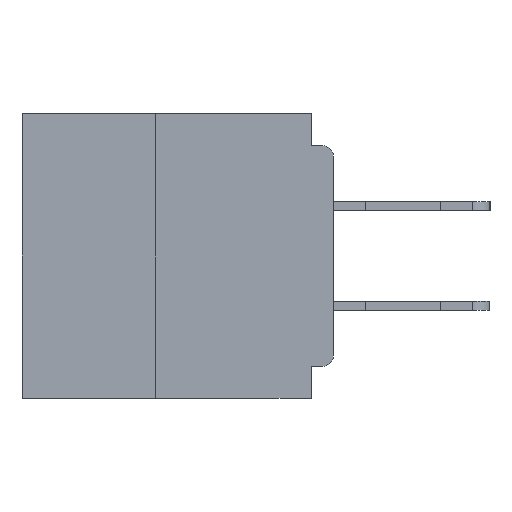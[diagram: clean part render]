
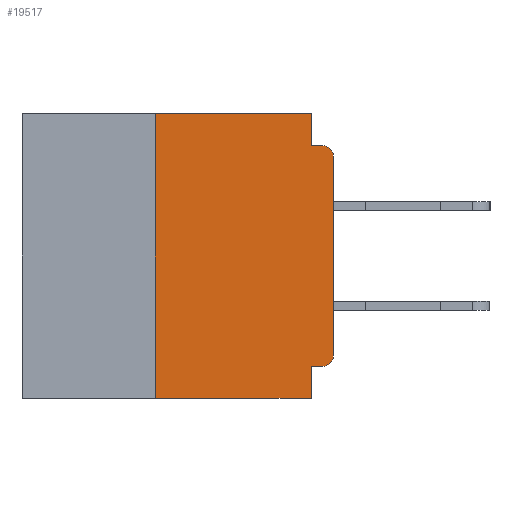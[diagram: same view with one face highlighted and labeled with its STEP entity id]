
A CAD part, left-side view. The second image highlights one B-rep face of the part: STEP entity #19517.
In plain terms, the highlighted planar face has unit normal (-1, 0, 0).
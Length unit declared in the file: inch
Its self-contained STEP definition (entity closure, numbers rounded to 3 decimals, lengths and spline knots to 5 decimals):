
#473 = EDGE_CURVE ( 'NONE', #25092, #37053, #29028, .T. ) ;
#1003 = ORIENTED_EDGE ( 'NONE', *, *, #13540, .F. ) ;
#2314 = VERTEX_POINT ( 'NONE', #25196 ) ;
#2443 = LINE ( 'NONE', #6597, #16447 ) ;
#2663 = EDGE_CURVE ( 'NONE', #30308, #9962, #35684, .T. ) ;
#3345 = DIRECTION ( 'NONE',  ( 0., 0., -1. ) ) ;
#3607 = ORIENTED_EDGE ( 'NONE', *, *, #13655, .T. ) ;
#4194 = VECTOR ( 'NONE', #34065, 39.37008 ) ;
#6597 = CARTESIAN_POINT ( 'NONE',  ( 0., 0.031, 0. ) ) ;
#7806 = CARTESIAN_POINT ( 'NONE',  ( 0., 0.25, -0.4 ) ) ;
#8055 = DIRECTION ( 'NONE',  ( 0., 0., 1. ) ) ;
#9294 = CARTESIAN_POINT ( 'NONE',  ( 0., 0.015, -0.045 ) ) ;
#9733 = ORIENTED_EDGE ( 'NONE', *, *, #35837, .F. ) ;
#9962 = VERTEX_POINT ( 'NONE', #22703 ) ;
#10027 = DIRECTION ( 'NONE',  ( 0., 0., -1. ) ) ;
#11047 = ORIENTED_EDGE ( 'NONE', *, *, #473, .F. ) ;
#12181 = EDGE_CURVE ( 'NONE', #35895, #25092, #21836, .T. ) ;
#12906 = DIRECTION ( 'NONE',  ( -1., 0., 0. ) ) ;
#12937 = FACE_OUTER_BOUND ( 'NONE', #22376, .T. ) ;
#13441 = LINE ( 'NONE', #34548, #27325 ) ;
#13540 = EDGE_CURVE ( 'NONE', #9962, #2314, #29599, .T. ) ;
#13655 = EDGE_CURVE ( 'NONE', #30308, #34135, #25893, .T. ) ;
#13798 = LINE ( 'NONE', #23938, #36373 ) ;
#13968 = VECTOR ( 'NONE', #19713, 39.37008 ) ;
#14230 = ORIENTED_EDGE ( 'NONE', *, *, #12181, .F. ) ;
#14853 = CARTESIAN_POINT ( 'NONE',  ( 0., 0.25, -0.4 ) ) ;
#15555 = ORIENTED_EDGE ( 'NONE', *, *, #24745, .T. ) ;
#16095 = ORIENTED_EDGE ( 'NONE', *, *, #35949, .T. ) ;
#16445 = CARTESIAN_POINT ( 'NONE',  ( 0., 0.015, -0.34 ) ) ;
#16447 = VECTOR ( 'NONE', #24414, 39.37008 ) ;
#17459 = LINE ( 'NONE', #32330, #32308 ) ;
#17698 = VERTEX_POINT ( 'NONE', #9294 ) ;
#17785 = CARTESIAN_POINT ( 'NONE',  ( 0., 0., -0.34 ) ) ;
#18180 = CARTESIAN_POINT ( 'NONE',  ( 0., 0.437, 0. ) ) ;
#18239 = CARTESIAN_POINT ( 'NONE',  ( 0., 0.015, -0.355 ) ) ;
#18323 = VERTEX_POINT ( 'NONE', #35823 ) ;
#18582 = ORIENTED_EDGE ( 'NONE', *, *, #37775, .F. ) ;
#19431 = DIRECTION ( 'NONE',  ( 0., 0., -1. ) ) ;
#19517 = ADVANCED_FACE ( 'NONE', ( #12937 ), #35854, .F. ) ;
#19713 = DIRECTION ( 'NONE',  ( 0., 0., 1. ) ) ;
#20894 = ORIENTED_EDGE ( 'NONE', *, *, #2663, .F. ) ;
#21199 = DIRECTION ( 'NONE',  ( 1., 0., 0. ) ) ;
#21380 = CIRCLE ( 'NONE', #37901, 0.015 ) ;
#21836 = LINE ( 'NONE', #7806, #13968 ) ;
#22376 = EDGE_LOOP ( 'NONE', ( #27587, #15555, #9733, #18582, #11047, #14230, #16095, #1003, #20894, #3607 ) ) ;
#22656 = VECTOR ( 'NONE', #10027, 39.37008 ) ;
#22703 = CARTESIAN_POINT ( 'NONE',  ( 0., 0.031, -0.355 ) ) ;
#23833 = CARTESIAN_POINT ( 'NONE',  ( 0., 0.031, 0. ) ) ;
#23938 = CARTESIAN_POINT ( 'NONE',  ( 0., 0.437, -0.4 ) ) ;
#24414 = DIRECTION ( 'NONE',  ( 0., 0., -1. ) ) ;
#24745 = EDGE_CURVE ( 'NONE', #37176, #17698, #21380, .T. ) ;
#25092 = VERTEX_POINT ( 'NONE', #26100 ) ;
#25196 = CARTESIAN_POINT ( 'NONE',  ( 0., 0.031, -0.4 ) ) ;
#25893 = CIRCLE ( 'NONE', #33988, 0.015 ) ;
#26100 = CARTESIAN_POINT ( 'NONE',  ( 0., 0.25, 0. ) ) ;
#27157 = VECTOR ( 'NONE', #32456, 39.37008 ) ;
#27325 = VECTOR ( 'NONE', #8055, 39.37008 ) ;
#27535 = AXIS2_PLACEMENT_3D ( 'NONE', #18180, #21199, #3345 ) ;
#27587 = ORIENTED_EDGE ( 'NONE', *, *, #29976, .T. ) ;
#27757 = CARTESIAN_POINT ( 'NONE',  ( 0., 0.031, -0.4 ) ) ;
#28556 = CARTESIAN_POINT ( 'NONE',  ( 0., 0., -0.355 ) ) ;
#29028 = LINE ( 'NONE', #31839, #27157 ) ;
#29493 = DIRECTION ( 'NONE',  ( 0., -1., 0. ) ) ;
#29599 = LINE ( 'NONE', #27757, #22656 ) ;
#29976 = EDGE_CURVE ( 'NONE', #34135, #37176, #13441, .T. ) ;
#30308 = VERTEX_POINT ( 'NONE', #18239 ) ;
#30626 = CARTESIAN_POINT ( 'NONE',  ( 0., 0.015, -0.06 ) ) ;
#31839 = CARTESIAN_POINT ( 'NONE',  ( 0., 0.437, 0. ) ) ;
#32308 = VECTOR ( 'NONE', #29493, 39.37008 ) ;
#32330 = CARTESIAN_POINT ( 'NONE',  ( 0., 0., -0.045 ) ) ;
#32456 = DIRECTION ( 'NONE',  ( 0., -1., 0. ) ) ;
#33206 = CARTESIAN_POINT ( 'NONE',  ( 0., 0., -0.06 ) ) ;
#33566 = DIRECTION ( 'NONE',  ( 0., 0., -1. ) ) ;
#33988 = AXIS2_PLACEMENT_3D ( 'NONE', #16445, #37039, #19431 ) ;
#34065 = DIRECTION ( 'NONE',  ( 0., 1., 0. ) ) ;
#34135 = VERTEX_POINT ( 'NONE', #17785 ) ;
#34548 = CARTESIAN_POINT ( 'NONE',  ( 0., 0., 0. ) ) ;
#35684 = LINE ( 'NONE', #28556, #4194 ) ;
#35745 = DIRECTION ( 'NONE',  ( 0., -1., 0. ) ) ;
#35823 = CARTESIAN_POINT ( 'NONE',  ( 0., 0.031, -0.045 ) ) ;
#35837 = EDGE_CURVE ( 'NONE', #18323, #17698, #17459, .T. ) ;
#35854 = PLANE ( 'NONE',  #27535 ) ;
#35895 = VERTEX_POINT ( 'NONE', #14853 ) ;
#35949 = EDGE_CURVE ( 'NONE', #35895, #2314, #13798, .T. ) ;
#36373 = VECTOR ( 'NONE', #35745, 39.37008 ) ;
#37039 = DIRECTION ( 'NONE',  ( -1., 0., 0. ) ) ;
#37053 = VERTEX_POINT ( 'NONE', #23833 ) ;
#37176 = VERTEX_POINT ( 'NONE', #33206 ) ;
#37775 = EDGE_CURVE ( 'NONE', #37053, #18323, #2443, .T. ) ;
#37901 = AXIS2_PLACEMENT_3D ( 'NONE', #30626, #12906, #33566 ) ;
